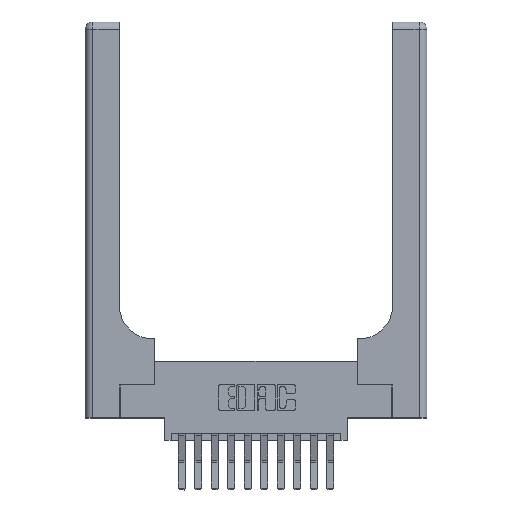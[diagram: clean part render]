
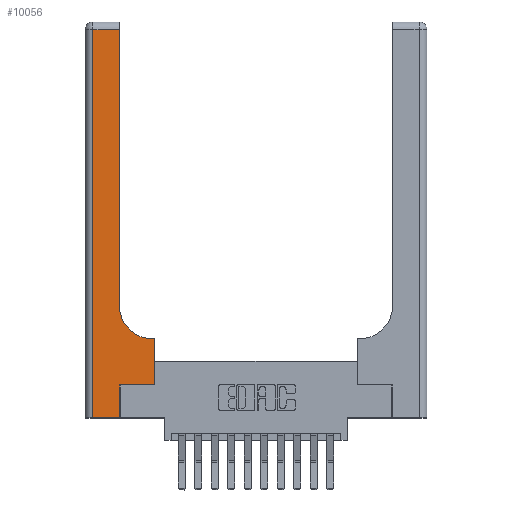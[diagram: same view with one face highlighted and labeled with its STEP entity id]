
A CAD part, top view. The second image highlights one B-rep face of the part: STEP entity #10056.
In plain terms, the highlighted planar face has unit normal (0, 0, 1).
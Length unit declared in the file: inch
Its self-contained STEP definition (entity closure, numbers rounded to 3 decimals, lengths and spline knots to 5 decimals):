
#197 = DIRECTION ( 'NONE',  ( 0., 1., 0. ) ) ;
#269 = ORIENTED_EDGE ( 'NONE', *, *, #15046, .T. ) ;
#773 = EDGE_CURVE ( 'NONE', #14770, #5732, #13420, .T. ) ;
#861 = ORIENTED_EDGE ( 'NONE', *, *, #773, .T. ) ;
#938 = EDGE_CURVE ( 'NONE', #13641, #12214, #4810, .T. ) ;
#978 = DIRECTION ( 'NONE',  ( -1., 0., 0. ) ) ;
#1078 = LINE ( 'NONE', #1154, #14087 ) ;
#1136 = DIRECTION ( 'NONE',  ( -1., 0., 0. ) ) ;
#1154 = CARTESIAN_POINT ( 'NONE',  ( 0.26, 0.6, 0.37 ) ) ;
#1245 = ORIENTED_EDGE ( 'NONE', *, *, #7595, .T. ) ;
#1598 = DIRECTION ( 'NONE',  ( 1., 0., 0. ) ) ;
#1776 = VERTEX_POINT ( 'NONE', #12419 ) ;
#1959 = CARTESIAN_POINT ( 'NONE',  ( 0.528, 0.25, 0.37 ) ) ;
#2645 = ORIENTED_EDGE ( 'NONE', *, *, #15991, .T. ) ;
#3062 = EDGE_CURVE ( 'NONE', #5997, #1776, #12591, .T. ) ;
#3553 = EDGE_CURVE ( 'NONE', #1776, #14923, #9703, .T. ) ;
#3669 = PLANE ( 'NONE',  #5840 ) ;
#3770 = VECTOR ( 'NONE', #9019, 39.37008 ) ;
#4810 = LINE ( 'NONE', #11809, #11480 ) ;
#5122 = VECTOR ( 'NONE', #1598, 39.37008 ) ;
#5732 = VERTEX_POINT ( 'NONE', #13433 ) ;
#5840 = AXIS2_PLACEMENT_3D ( 'NONE', #8697, #8791, #1136 ) ;
#5997 = VERTEX_POINT ( 'NONE', #12822 ) ;
#6291 = ORIENTED_EDGE ( 'NONE', *, *, #3553, .T. ) ;
#6310 = ORIENTED_EDGE ( 'NONE', *, *, #8816, .T. ) ;
#6348 = VECTOR ( 'NONE', #197, 39.37008 ) ;
#6801 = CARTESIAN_POINT ( 'NONE',  ( 0.06, 0., 0.37 ) ) ;
#7114 = ORIENTED_EDGE ( 'NONE', *, *, #938, .T. ) ;
#7552 = CARTESIAN_POINT ( 'NONE',  ( 0.51, 0.85, 0.37 ) ) ;
#7574 = DIRECTION ( 'NONE',  ( -1., 0., 0. ) ) ;
#7595 = EDGE_CURVE ( 'NONE', #5732, #10932, #8715, .T. ) ;
#7630 = CARTESIAN_POINT ( 'NONE',  ( 0.06, 2.94, 0.37 ) ) ;
#7784 = CARTESIAN_POINT ( 'NONE',  ( 0., 0., 0.37 ) ) ;
#7945 = VECTOR ( 'NONE', #8892, 39.37008 ) ;
#8076 = LINE ( 'NONE', #8639, #11376 ) ;
#8107 = DIRECTION ( 'NONE',  ( 0., 1., 0. ) ) ;
#8639 = CARTESIAN_POINT ( 'NONE',  ( 0., 2.94, 0.37 ) ) ;
#8697 = CARTESIAN_POINT ( 'NONE',  ( 0., 3., 0.37 ) ) ;
#8715 = LINE ( 'NONE', #8840, #7945 ) ;
#8789 = DIRECTION ( 'NONE',  ( 1., 0., 0. ) ) ;
#8791 = DIRECTION ( 'NONE',  ( 0., 0., -1. ) ) ;
#8816 = EDGE_CURVE ( 'NONE', #10932, #13641, #14666, .T. ) ;
#8840 = CARTESIAN_POINT ( 'NONE',  ( 0.265, 0., 0.37 ) ) ;
#8892 = DIRECTION ( 'NONE',  ( 0., 1., 0. ) ) ;
#9019 = DIRECTION ( 'NONE',  ( 1., 0., 0. ) ) ;
#9135 = CARTESIAN_POINT ( 'NONE',  ( 0.528, 0.6, 0.37 ) ) ;
#9484 = CARTESIAN_POINT ( 'NONE',  ( 0.06, 3., 0.37 ) ) ;
#9580 = CARTESIAN_POINT ( 'NONE',  ( 0.26, 2.94, 0.37 ) ) ;
#9703 = LINE ( 'NONE', #12777, #6348 ) ;
#10056 = ADVANCED_FACE ( 'NONE', ( #12184 ), #3669, .F. ) ;
#10509 = CARTESIAN_POINT ( 'NONE',  ( 0.265, 0.25, 0.37 ) ) ;
#10680 = DIRECTION ( 'NONE',  ( 0., -1., 0. ) ) ;
#10932 = VERTEX_POINT ( 'NONE', #13159 ) ;
#11376 = VECTOR ( 'NONE', #978, 39.37008 ) ;
#11480 = VECTOR ( 'NONE', #8107, 39.37008 ) ;
#11593 = ORIENTED_EDGE ( 'NONE', *, *, #13856, .T. ) ;
#11746 = VECTOR ( 'NONE', #10680, 39.37008 ) ;
#11809 = CARTESIAN_POINT ( 'NONE',  ( 0.528, 0.25, 0.37 ) ) ;
#11990 = ORIENTED_EDGE ( 'NONE', *, *, #3062, .T. ) ;
#12184 = FACE_OUTER_BOUND ( 'NONE', #15039, .T. ) ;
#12214 = VERTEX_POINT ( 'NONE', #9135 ) ;
#12419 = CARTESIAN_POINT ( 'NONE',  ( 0.26, 0.85, 0.37 ) ) ;
#12591 = CIRCLE ( 'NONE', #14797, 0.25 ) ;
#12777 = CARTESIAN_POINT ( 'NONE',  ( 0.26, 3., 0.37 ) ) ;
#12822 = CARTESIAN_POINT ( 'NONE',  ( 0.51, 0.6, 0.37 ) ) ;
#13159 = CARTESIAN_POINT ( 'NONE',  ( 0.265, 0.25, 0.37 ) ) ;
#13420 = LINE ( 'NONE', #7784, #3770 ) ;
#13433 = CARTESIAN_POINT ( 'NONE',  ( 0.265, 0., 0.37 ) ) ;
#13641 = VERTEX_POINT ( 'NONE', #1959 ) ;
#13856 = EDGE_CURVE ( 'NONE', #12214, #5997, #1078, .T. ) ;
#13880 = VERTEX_POINT ( 'NONE', #7630 ) ;
#14087 = VECTOR ( 'NONE', #7574, 39.37008 ) ;
#14666 = LINE ( 'NONE', #10509, #5122 ) ;
#14770 = VERTEX_POINT ( 'NONE', #6801 ) ;
#14797 = AXIS2_PLACEMENT_3D ( 'NONE', #7552, #16166, #8789 ) ;
#14923 = VERTEX_POINT ( 'NONE', #9580 ) ;
#14983 = LINE ( 'NONE', #9484, #11746 ) ;
#15039 = EDGE_LOOP ( 'NONE', ( #6291, #269, #2645, #861, #1245, #6310, #7114, #11593, #11990 ) ) ;
#15046 = EDGE_CURVE ( 'NONE', #14923, #13880, #8076, .T. ) ;
#15991 = EDGE_CURVE ( 'NONE', #13880, #14770, #14983, .T. ) ;
#16166 = DIRECTION ( 'NONE',  ( 0., 0., -1. ) ) ;
